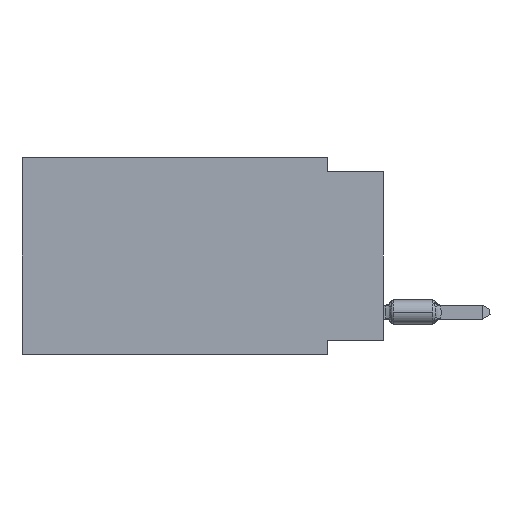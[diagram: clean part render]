
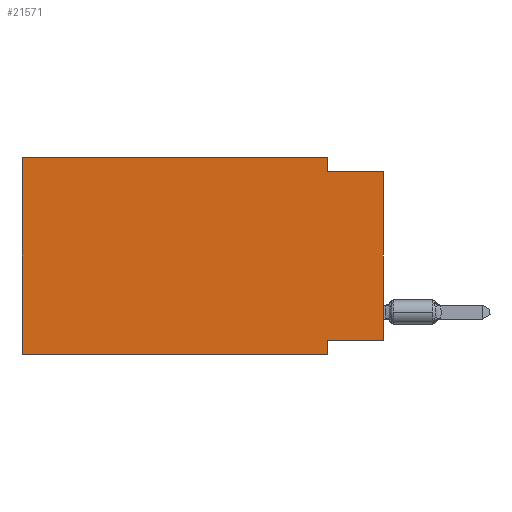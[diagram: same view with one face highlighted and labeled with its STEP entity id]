
A CAD part, left-side view. The second image highlights one B-rep face of the part: STEP entity #21571.
In plain terms, the highlighted planar face has unit normal (-1, 0, 0).
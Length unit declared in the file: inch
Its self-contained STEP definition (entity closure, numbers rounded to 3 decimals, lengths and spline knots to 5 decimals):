
#189 = VECTOR ( 'NONE', #11094, 39.37008 ) ;
#438 = ORIENTED_EDGE ( 'NONE', *, *, #20566, .F. ) ;
#2329 = ORIENTED_EDGE ( 'NONE', *, *, #4293, .F. ) ;
#3593 = CARTESIAN_POINT ( 'NONE',  ( 0., 0.645, 0. ) ) ;
#3777 = LINE ( 'NONE', #6206, #33781 ) ;
#3898 = FACE_OUTER_BOUND ( 'NONE', #29327, .T. ) ;
#4293 = EDGE_CURVE ( 'NONE', #24808, #6388, #3777, .T. ) ;
#4528 = DIRECTION ( 'NONE',  ( 0., 0., -1. ) ) ;
#4973 = CARTESIAN_POINT ( 'NONE',  ( 0., 0., -0.025 ) ) ;
#6048 = EDGE_CURVE ( 'NONE', #28179, #9953, #8154, .T. ) ;
#6206 = CARTESIAN_POINT ( 'NONE',  ( 0., 0.645, 0. ) ) ;
#6351 = VERTEX_POINT ( 'NONE', #10524 ) ;
#6378 = ORIENTED_EDGE ( 'NONE', *, *, #6048, .F. ) ;
#6388 = VERTEX_POINT ( 'NONE', #23368 ) ;
#6401 = ORIENTED_EDGE ( 'NONE', *, *, #35929, .F. ) ;
#6800 = DIRECTION ( 'NONE',  ( 0., 0., 1. ) ) ;
#7902 = DIRECTION ( 'NONE',  ( 0., 0., 1. ) ) ;
#8055 = CARTESIAN_POINT ( 'NONE',  ( 0., 0.1, -0.35 ) ) ;
#8154 = LINE ( 'NONE', #26238, #30667 ) ;
#9690 = VECTOR ( 'NONE', #15859, 39.37008 ) ;
#9953 = VERTEX_POINT ( 'NONE', #15997 ) ;
#10183 = DIRECTION ( 'NONE',  ( 0., -1., 0. ) ) ;
#10365 = VECTOR ( 'NONE', #12273, 39.37008 ) ;
#10524 = CARTESIAN_POINT ( 'NONE',  ( 0., 0., -0.325 ) ) ;
#10679 = DIRECTION ( 'NONE',  ( 0., 0., -1. ) ) ;
#10822 = ORIENTED_EDGE ( 'NONE', *, *, #34390, .F. ) ;
#10859 = ORIENTED_EDGE ( 'NONE', *, *, #17895, .F. ) ;
#11094 = DIRECTION ( 'NONE',  ( 0., 1., 0. ) ) ;
#11655 = VECTOR ( 'NONE', #7902, 39.37008 ) ;
#12248 = VERTEX_POINT ( 'NONE', #21610 ) ;
#12273 = DIRECTION ( 'NONE',  ( 0., -1., 0. ) ) ;
#13832 = AXIS2_PLACEMENT_3D ( 'NONE', #16166, #38232, #10679 ) ;
#15859 = DIRECTION ( 'NONE',  ( 0., -1., 0. ) ) ;
#15872 = VECTOR ( 'NONE', #23102, 39.37008 ) ;
#15997 = CARTESIAN_POINT ( 'NONE',  ( 0., 0.1, -0.025 ) ) ;
#16166 = CARTESIAN_POINT ( 'NONE',  ( 0., 0.645, 0. ) ) ;
#17708 = VERTEX_POINT ( 'NONE', #27188 ) ;
#17895 = EDGE_CURVE ( 'NONE', #12248, #17708, #29364, .T. ) ;
#19907 = CARTESIAN_POINT ( 'NONE',  ( 0., 0.1, 0. ) ) ;
#20566 = EDGE_CURVE ( 'NONE', #6388, #28179, #31149, .T. ) ;
#21571 = ADVANCED_FACE ( 'NONE', ( #3898 ), #26153, .F. ) ;
#21610 = CARTESIAN_POINT ( 'NONE',  ( 0., 0.1, -0.325 ) ) ;
#23102 = DIRECTION ( 'NONE',  ( 0., 0., -1. ) ) ;
#23368 = CARTESIAN_POINT ( 'NONE',  ( 0., 0.645, 0. ) ) ;
#24808 = VERTEX_POINT ( 'NONE', #26077 ) ;
#25308 = EDGE_CURVE ( 'NONE', #6351, #26070, #35233, .T. ) ;
#26070 = VERTEX_POINT ( 'NONE', #4973 ) ;
#26077 = CARTESIAN_POINT ( 'NONE',  ( 0., 0.645, -0.35 ) ) ;
#26153 = PLANE ( 'NONE',  #13832 ) ;
#26238 = CARTESIAN_POINT ( 'NONE',  ( 0., 0.1, 0. ) ) ;
#27188 = CARTESIAN_POINT ( 'NONE',  ( 0., 0.1, -0.35 ) ) ;
#28104 = CARTESIAN_POINT ( 'NONE',  ( 0., 0.645, -0.35 ) ) ;
#28157 = CARTESIAN_POINT ( 'NONE',  ( 0., 0., -0.025 ) ) ;
#28179 = VERTEX_POINT ( 'NONE', #19907 ) ;
#29327 = EDGE_LOOP ( 'NONE', ( #34537, #10822, #6378, #438, #2329, #35156, #10859, #6401 ) ) ;
#29364 = LINE ( 'NONE', #8055, #15872 ) ;
#29671 = VECTOR ( 'NONE', #10183, 39.37008 ) ;
#30667 = VECTOR ( 'NONE', #4528, 39.37008 ) ;
#31149 = LINE ( 'NONE', #3593, #9690 ) ;
#32016 = CARTESIAN_POINT ( 'NONE',  ( 0., 0., 0. ) ) ;
#32613 = LINE ( 'NONE', #38646, #189 ) ;
#33151 = EDGE_CURVE ( 'NONE', #24808, #17708, #34529, .T. ) ;
#33781 = VECTOR ( 'NONE', #6800, 39.37008 ) ;
#34390 = EDGE_CURVE ( 'NONE', #9953, #26070, #36818, .T. ) ;
#34529 = LINE ( 'NONE', #28104, #29671 ) ;
#34537 = ORIENTED_EDGE ( 'NONE', *, *, #25308, .T. ) ;
#35156 = ORIENTED_EDGE ( 'NONE', *, *, #33151, .T. ) ;
#35233 = LINE ( 'NONE', #32016, #11655 ) ;
#35929 = EDGE_CURVE ( 'NONE', #6351, #12248, #32613, .T. ) ;
#36818 = LINE ( 'NONE', #28157, #10365 ) ;
#38232 = DIRECTION ( 'NONE',  ( 1., 0., 0. ) ) ;
#38646 = CARTESIAN_POINT ( 'NONE',  ( 0., 0., -0.325 ) ) ;
